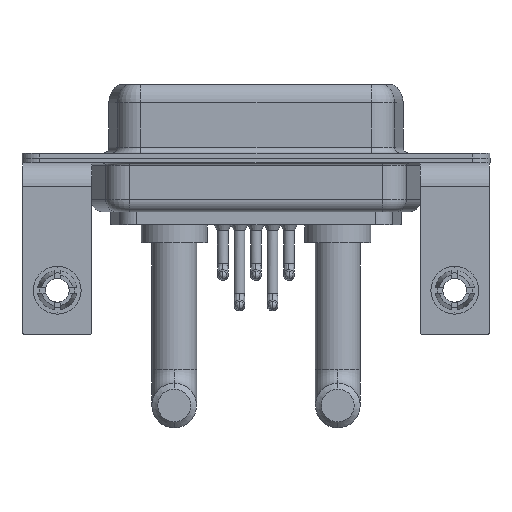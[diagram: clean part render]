
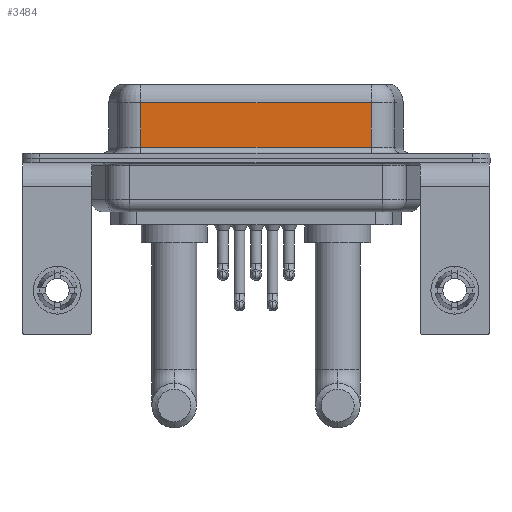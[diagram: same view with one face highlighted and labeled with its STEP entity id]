
A CAD part, front view. The second image highlights one B-rep face of the part: STEP entity #3484.
In plain terms, the highlighted planar face has unit normal (0, -1, 0).
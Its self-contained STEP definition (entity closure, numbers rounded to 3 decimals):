
#299 = VECTOR ( 'NONE', #12139, 1000. ) ;
#551 = CARTESIAN_POINT ( 'NONE',  ( 26.287, -3.95, 6.4 ) ) ;
#836 = CARTESIAN_POINT ( 'NONE',  ( 7.013, -3.95, 6.4 ) ) ;
#1072 = ORIENTED_EDGE ( 'NONE', *, *, #8213, .T. ) ;
#1588 = VECTOR ( 'NONE', #12848, 1000. ) ;
#2005 = PLANE ( 'NONE',  #6434 ) ;
#2369 = ORIENTED_EDGE ( 'NONE', *, *, #7487, .F. ) ;
#2782 = EDGE_LOOP ( 'NONE', ( #2369, #16490, #9784, #1072 ) ) ;
#3484 = ADVANCED_FACE ( 'NONE', ( #4951 ), #2005, .F. ) ;
#3906 = CARTESIAN_POINT ( 'NONE',  ( 26.287, -3.95, 0.9 ) ) ;
#3910 = DIRECTION ( 'NONE',  ( 0., 0., -1. ) ) ;
#4951 = FACE_OUTER_BOUND ( 'NONE', #2782, .T. ) ;
#4966 = VECTOR ( 'NONE', #3910, 1000. ) ;
#6434 = AXIS2_PLACEMENT_3D ( 'NONE', #551, #13611, #6512 ) ;
#6512 = DIRECTION ( 'NONE',  ( 0., 0., 1. ) ) ;
#7487 = EDGE_CURVE ( 'NONE', #14359, #15827, #14233, .T. ) ;
#8213 = EDGE_CURVE ( 'NONE', #9018, #15827, #11850, .T. ) ;
#9018 = VERTEX_POINT ( 'NONE', #13083 ) ;
#9776 = VERTEX_POINT ( 'NONE', #10964 ) ;
#9784 = ORIENTED_EDGE ( 'NONE', *, *, #9788, .T. ) ;
#9788 = EDGE_CURVE ( 'NONE', #9776, #9018, #14276, .T. ) ;
#9923 = CARTESIAN_POINT ( 'NONE',  ( 26.287, -3.95, 4.65 ) ) ;
#10964 = CARTESIAN_POINT ( 'NONE',  ( 7.013, -3.95, 4.65 ) ) ;
#11041 = EDGE_CURVE ( 'NONE', #14359, #9776, #15654, .T. ) ;
#11850 = LINE ( 'NONE', #17797, #299 ) ;
#12139 = DIRECTION ( 'NONE',  ( 1., 0., 0. ) ) ;
#12526 = DIRECTION ( 'NONE',  ( 0., 0., -1. ) ) ;
#12848 = DIRECTION ( 'NONE',  ( -1., 0., 0. ) ) ;
#13083 = CARTESIAN_POINT ( 'NONE',  ( 7.013, -3.95, 0.9 ) ) ;
#13611 = DIRECTION ( 'NONE',  ( 0., 1., 0. ) ) ;
#14233 = LINE ( 'NONE', #15492, #4966 ) ;
#14276 = LINE ( 'NONE', #836, #15228 ) ;
#14359 = VERTEX_POINT ( 'NONE', #14387 ) ;
#14387 = CARTESIAN_POINT ( 'NONE',  ( 26.287, -3.95, 4.65 ) ) ;
#15228 = VECTOR ( 'NONE', #12526, 1000. ) ;
#15492 = CARTESIAN_POINT ( 'NONE',  ( 26.287, -3.95, 6.4 ) ) ;
#15654 = LINE ( 'NONE', #9923, #1588 ) ;
#15827 = VERTEX_POINT ( 'NONE', #3906 ) ;
#16490 = ORIENTED_EDGE ( 'NONE', *, *, #11041, .T. ) ;
#17797 = CARTESIAN_POINT ( 'NONE',  ( 26.287, -3.95, 0.9 ) ) ;
